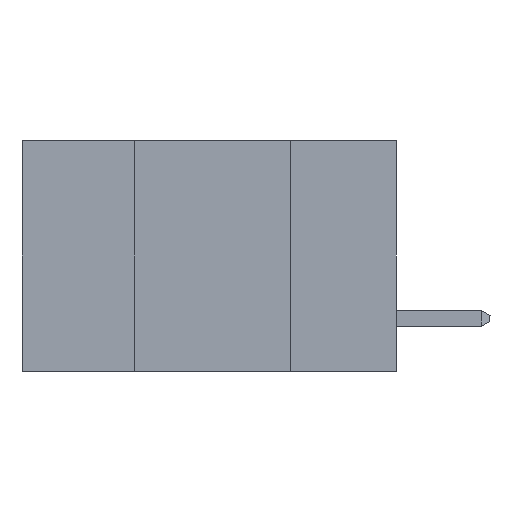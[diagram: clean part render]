
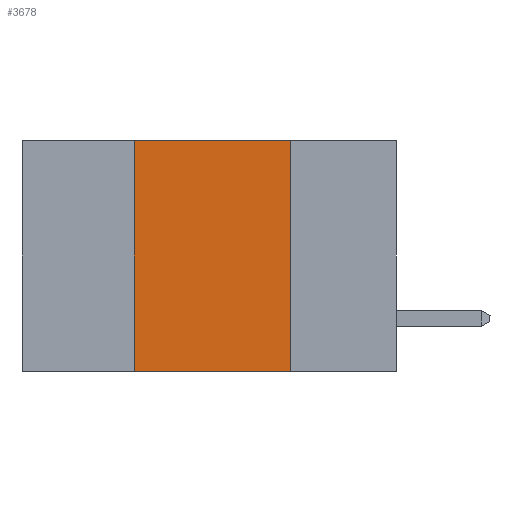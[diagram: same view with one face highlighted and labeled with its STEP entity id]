
A CAD part, left-side view. The second image highlights one B-rep face of the part: STEP entity #3678.
In plain terms, the highlighted planar face has unit normal (-1, 0, 0).
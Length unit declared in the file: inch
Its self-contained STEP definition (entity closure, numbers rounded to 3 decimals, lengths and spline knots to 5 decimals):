
#433 = FACE_OUTER_BOUND ( 'NONE', #4452, .T. ) ;
#592 = EDGE_CURVE ( 'NONE', #5239, #5634, #6781, .T. ) ;
#694 = CARTESIAN_POINT ( 'NONE',  ( 0., 0.6, -0.37 ) ) ;
#1059 = LINE ( 'NONE', #12951, #19248 ) ;
#1650 = ORIENTED_EDGE ( 'NONE', *, *, #10020, .F. ) ;
#2832 = CARTESIAN_POINT ( 'NONE',  ( 0., 0.42, 0. ) ) ;
#3476 = EDGE_CURVE ( 'NONE', #4143, #5239, #10546, .T. ) ;
#3603 = DIRECTION ( 'NONE',  ( 1., 0., 0. ) ) ;
#3678 = ADVANCED_FACE ( 'NONE', ( #433 ), #8355, .F. ) ;
#3851 = CARTESIAN_POINT ( 'NONE',  ( 0., 0.17, 0. ) ) ;
#4143 = VERTEX_POINT ( 'NONE', #2832 ) ;
#4452 = EDGE_LOOP ( 'NONE', ( #15251, #6930, #1650, #12244 ) ) ;
#5239 = VERTEX_POINT ( 'NONE', #3851 ) ;
#5634 = VERTEX_POINT ( 'NONE', #18598 ) ;
#6781 = LINE ( 'NONE', #9850, #7823 ) ;
#6930 = ORIENTED_EDGE ( 'NONE', *, *, #3476, .F. ) ;
#7823 = VECTOR ( 'NONE', #15600, 39.37008 ) ;
#8355 = PLANE ( 'NONE',  #10381 ) ;
#9020 = VECTOR ( 'NONE', #9255, 39.37008 ) ;
#9255 = DIRECTION ( 'NONE',  ( 0., -1., 0. ) ) ;
#9564 = VERTEX_POINT ( 'NONE', #11575 ) ;
#9850 = CARTESIAN_POINT ( 'NONE',  ( 0., 0.17, -0.37 ) ) ;
#10020 = EDGE_CURVE ( 'NONE', #9564, #4143, #1059, .T. ) ;
#10381 = AXIS2_PLACEMENT_3D ( 'NONE', #11026, #3603, #17276 ) ;
#10546 = LINE ( 'NONE', #15294, #9020 ) ;
#11026 = CARTESIAN_POINT ( 'NONE',  ( 0., 0.6, 0. ) ) ;
#11575 = CARTESIAN_POINT ( 'NONE',  ( 0., 0.42, -0.37 ) ) ;
#12244 = ORIENTED_EDGE ( 'NONE', *, *, #14400, .T. ) ;
#12786 = LINE ( 'NONE', #694, #16203 ) ;
#12951 = CARTESIAN_POINT ( 'NONE',  ( 0., 0.42, -0.37 ) ) ;
#14400 = EDGE_CURVE ( 'NONE', #9564, #5634, #12786, .T. ) ;
#14917 = DIRECTION ( 'NONE',  ( 0., 0., 1. ) ) ;
#15251 = ORIENTED_EDGE ( 'NONE', *, *, #592, .F. ) ;
#15294 = CARTESIAN_POINT ( 'NONE',  ( 0., 0.6, 0. ) ) ;
#15600 = DIRECTION ( 'NONE',  ( 0., 0., -1. ) ) ;
#16203 = VECTOR ( 'NONE', #17544, 39.37008 ) ;
#17276 = DIRECTION ( 'NONE',  ( 0., 0., -1. ) ) ;
#17544 = DIRECTION ( 'NONE',  ( 0., -1., 0. ) ) ;
#18598 = CARTESIAN_POINT ( 'NONE',  ( 0., 0.17, -0.37 ) ) ;
#19248 = VECTOR ( 'NONE', #14917, 39.37008 ) ;
